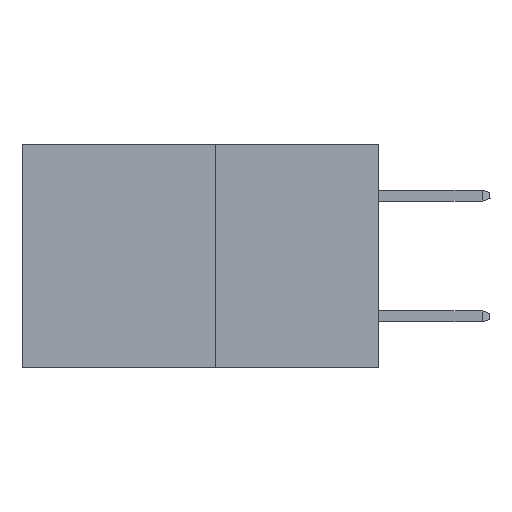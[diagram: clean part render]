
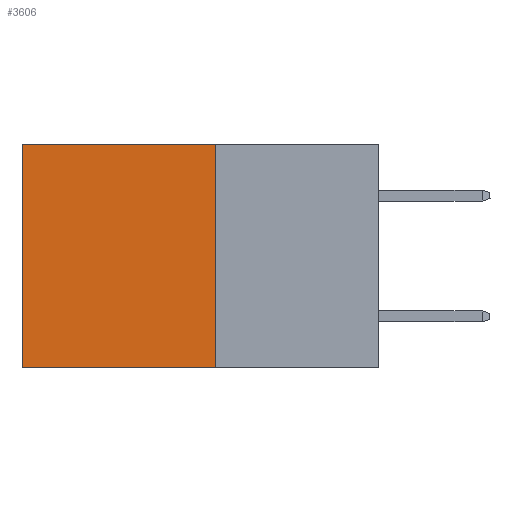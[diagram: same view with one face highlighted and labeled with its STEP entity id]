
A CAD part, left-side view. The second image highlights one B-rep face of the part: STEP entity #3606.
In plain terms, the highlighted planar face has unit normal (-1, 0, 0).
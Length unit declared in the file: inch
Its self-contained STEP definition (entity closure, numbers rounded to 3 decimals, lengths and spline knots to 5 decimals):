
#104 = CARTESIAN_POINT ( 'NONE',  ( 0.277, 0.59, -0.37 ) ) ;
#128 = VECTOR ( 'NONE', #14154, 39.37008 ) ;
#557 = DIRECTION ( 'NONE',  ( 0., 0., -1. ) ) ;
#703 = DIRECTION ( 'NONE',  ( 1., 0., 0. ) ) ;
#1164 = FACE_OUTER_BOUND ( 'NONE', #22188, .T. ) ;
#1629 = CARTESIAN_POINT ( 'NONE',  ( 0.277, 0.27, -0.37 ) ) ;
#2317 = VERTEX_POINT ( 'NONE', #21407 ) ;
#3393 = ORIENTED_EDGE ( 'NONE', *, *, #17046, .F. ) ;
#3606 = ADVANCED_FACE ( 'NONE', ( #1164 ), #9650, .F. ) ;
#3841 = CARTESIAN_POINT ( 'NONE',  ( 0.277, 0.59, -0.37 ) ) ;
#4187 = ORIENTED_EDGE ( 'NONE', *, *, #22273, .T. ) ;
#4824 = VERTEX_POINT ( 'NONE', #104 ) ;
#5578 = DIRECTION ( 'NONE',  ( 0., 0., -1. ) ) ;
#8553 = CARTESIAN_POINT ( 'NONE',  ( 0.277, 0.27, -0.37 ) ) ;
#8867 = AXIS2_PLACEMENT_3D ( 'NONE', #13181, #703, #13256 ) ;
#9449 = LINE ( 'NONE', #3841, #23030 ) ;
#9650 = PLANE ( 'NONE',  #8867 ) ;
#9877 = VECTOR ( 'NONE', #557, 39.37008 ) ;
#12010 = CARTESIAN_POINT ( 'NONE',  ( 0.277, 0.27, 0. ) ) ;
#12215 = EDGE_CURVE ( 'NONE', #17142, #4824, #9449, .T. ) ;
#13038 = CARTESIAN_POINT ( 'NONE',  ( 0.277, 0.27, -0.37 ) ) ;
#13181 = CARTESIAN_POINT ( 'NONE',  ( 0.277, 0.27, -0.37 ) ) ;
#13256 = DIRECTION ( 'NONE',  ( 0., 0., -1. ) ) ;
#14154 = DIRECTION ( 'NONE',  ( 0., 1., 0. ) ) ;
#14616 = LINE ( 'NONE', #13038, #9877 ) ;
#16105 = VERTEX_POINT ( 'NONE', #8553 ) ;
#17046 = EDGE_CURVE ( 'NONE', #16105, #4824, #18028, .T. ) ;
#17070 = VECTOR ( 'NONE', #20863, 39.37008 ) ;
#17142 = VERTEX_POINT ( 'NONE', #19620 ) ;
#17624 = LINE ( 'NONE', #12010, #17070 ) ;
#18028 = LINE ( 'NONE', #1629, #128 ) ;
#18867 = ORIENTED_EDGE ( 'NONE', *, *, #12215, .T. ) ;
#19620 = CARTESIAN_POINT ( 'NONE',  ( 0.277, 0.59, 0. ) ) ;
#20863 = DIRECTION ( 'NONE',  ( 0., 1., 0. ) ) ;
#21284 = EDGE_CURVE ( 'NONE', #2317, #16105, #14616, .T. ) ;
#21407 = CARTESIAN_POINT ( 'NONE',  ( 0.277, 0.27, 0. ) ) ;
#22188 = EDGE_LOOP ( 'NONE', ( #18867, #3393, #22963, #4187 ) ) ;
#22273 = EDGE_CURVE ( 'NONE', #2317, #17142, #17624, .T. ) ;
#22963 = ORIENTED_EDGE ( 'NONE', *, *, #21284, .F. ) ;
#23030 = VECTOR ( 'NONE', #5578, 39.37008 ) ;
